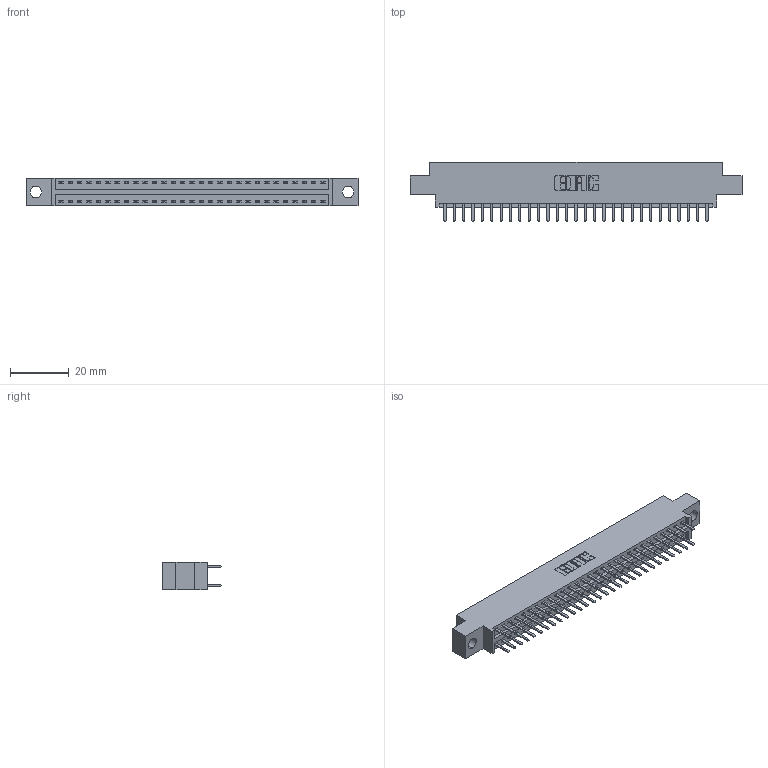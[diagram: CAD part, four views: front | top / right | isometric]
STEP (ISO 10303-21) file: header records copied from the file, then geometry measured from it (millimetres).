
FILE_DESCRIPTION (( 'STEP AP203' ), '1' );
FILE_NAME ('396-058-520-804.STEP', '2018-09-08T10:52:59', ( '' ), ( '' ), 'SwSTEP 2.0', 'SolidWorks 2016', '' );
FILE_SCHEMA (( 'CONFIG_CONTROL_DESIGN' ));
Length unit declared in the file: inch
Products named in the file (3): 345-292-001_345-293-120; 396-058-520-804; 346 Part_0.170 Offset - 0.156 Dia-TH
Assembly tree (59 placements, depth 2):
  396-058-520-804
    346 Part_0.170 Offset - 0.156 Dia-TH
    345-292-001_345-293-120  x58
Bounding box: 112.65 x 20.02 x 9.4 mm (x, y, z)
Volume: 10615.7 mm3; surface area: 14321 mm2
Topology: 59 solids, 59 shells, 3374 faces, 9795 edges, 6374 vertices
Faces by surface type: plane 2226, cylinder 1148
Entity records: 20925 total; most frequent: CARTESIAN_POINT 3480, ORIENTED_EDGE 3402, DIRECTION 3105, EDGE_CURVE 1701, VECTOR 1449, LINE 1449, VERTEX_POINT 1130, AXIS2_PLACEMENT_3D 828
